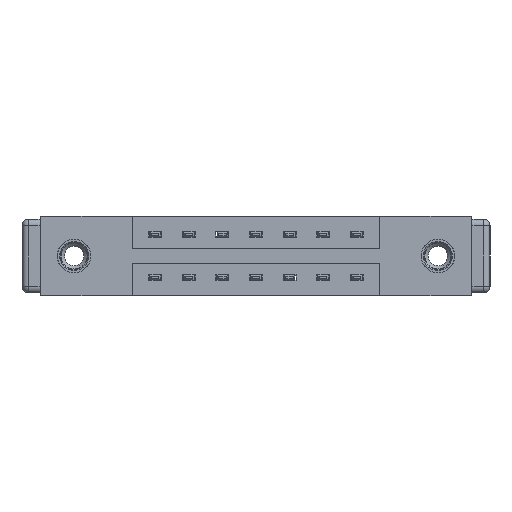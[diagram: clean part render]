
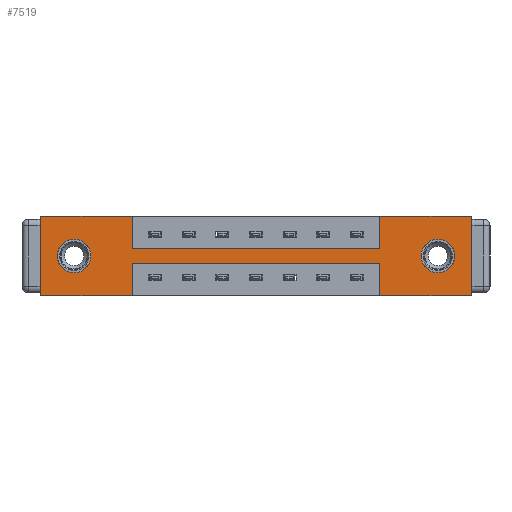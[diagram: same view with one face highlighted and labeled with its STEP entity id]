
A CAD part, front view. The second image highlights one B-rep face of the part: STEP entity #7519.
In plain terms, the highlighted planar face has unit normal (0, -1, 0).
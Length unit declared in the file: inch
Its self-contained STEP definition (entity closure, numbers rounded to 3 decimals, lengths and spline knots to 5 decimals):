
#92 = EDGE_CURVE ( 'NONE', #5666, #3161, #3983, .T. ) ;
#186 = CARTESIAN_POINT ( 'NONE',  ( 0.155, 0., -0.185 ) ) ;
#267 = CARTESIAN_POINT ( 'NONE',  ( 1.843, 0., -0.185 ) ) ;
#379 = VECTOR ( 'NONE', #10934, 39.37008 ) ;
#504 = VECTOR ( 'NONE', #2358, 39.37008 ) ;
#543 = CIRCLE ( 'NONE', #1455, 0.078 ) ;
#605 = CARTESIAN_POINT ( 'NONE',  ( 0.155, 0., -0.107 ) ) ;
#740 = CARTESIAN_POINT ( 'NONE',  ( 0., 0., 0. ) ) ;
#781 = FACE_BOUND ( 'NONE', #3398, .T. ) ;
#900 = ORIENTED_EDGE ( 'NONE', *, *, #6440, .F. ) ;
#1031 = DIRECTION ( 'NONE',  ( -1., 0., 0. ) ) ;
#1211 = DIRECTION ( 'NONE',  ( 0., 0., -1. ) ) ;
#1355 = CARTESIAN_POINT ( 'NONE',  ( 0.425, 0., -0.37 ) ) ;
#1396 = VERTEX_POINT ( 'NONE', #8295 ) ;
#1453 = CARTESIAN_POINT ( 'NONE',  ( 1.998, 0., -0.37 ) ) ;
#1455 = AXIS2_PLACEMENT_3D ( 'NONE', #186, #8013, #8932 ) ;
#1549 = EDGE_CURVE ( 'NONE', #3890, #11087, #4889, .T. ) ;
#1707 = CARTESIAN_POINT ( 'NONE',  ( 0., 0., -0.37 ) ) ;
#1768 = LINE ( 'NONE', #12552, #2092 ) ;
#1771 = DIRECTION ( 'NONE',  ( 0., 1., 0. ) ) ;
#1783 = CIRCLE ( 'NONE', #2567, 0.078 ) ;
#1805 = EDGE_CURVE ( 'NONE', #6223, #1396, #12031, .T. ) ;
#1850 = DIRECTION ( 'NONE',  ( 0., 0., -1. ) ) ;
#2052 = DIRECTION ( 'NONE',  ( 0., 0., 1. ) ) ;
#2061 = ORIENTED_EDGE ( 'NONE', *, *, #7285, .F. ) ;
#2092 = VECTOR ( 'NONE', #5840, 39.37008 ) ;
#2126 = VECTOR ( 'NONE', #8789, 39.37008 ) ;
#2205 = CARTESIAN_POINT ( 'NONE',  ( 0.425, 0., -0.37 ) ) ;
#2211 = DIRECTION ( 'NONE',  ( 0., 1., 0. ) ) ;
#2242 = EDGE_CURVE ( 'NONE', #11909, #10411, #7346, .T. ) ;
#2358 = DIRECTION ( 'NONE',  ( 0., 0., -1. ) ) ;
#2479 = LINE ( 'NONE', #7652, #12472 ) ;
#2567 = AXIS2_PLACEMENT_3D ( 'NONE', #3620, #1771, #10451 ) ;
#2671 = AXIS2_PLACEMENT_3D ( 'NONE', #267, #6084, #1211 ) ;
#2679 = AXIS2_PLACEMENT_3D ( 'NONE', #11857, #2211, #5115 ) ;
#2734 = ORIENTED_EDGE ( 'NONE', *, *, #5673, .F. ) ;
#2827 = PLANE ( 'NONE',  #10467 ) ;
#3148 = VERTEX_POINT ( 'NONE', #11028 ) ;
#3161 = VERTEX_POINT ( 'NONE', #1453 ) ;
#3244 = CARTESIAN_POINT ( 'NONE',  ( 0., 0., 0. ) ) ;
#3254 = LINE ( 'NONE', #8975, #8152 ) ;
#3398 = EDGE_LOOP ( 'NONE', ( #8268, #8948 ) ) ;
#3434 = LINE ( 'NONE', #6838, #6486 ) ;
#3491 = CARTESIAN_POINT ( 'NONE',  ( 0.425, 0., -0.22 ) ) ;
#3609 = ORIENTED_EDGE ( 'NONE', *, *, #4107, .F. ) ;
#3620 = CARTESIAN_POINT ( 'NONE',  ( 0.155, 0., -0.185 ) ) ;
#3704 = LINE ( 'NONE', #9032, #11931 ) ;
#3890 = VERTEX_POINT ( 'NONE', #3244 ) ;
#3904 = CARTESIAN_POINT ( 'NONE',  ( 0.425, 0., -0.22 ) ) ;
#3905 = CARTESIAN_POINT ( 'NONE',  ( 0.155, 0., -0.263 ) ) ;
#3983 = LINE ( 'NONE', #12521, #8166 ) ;
#4000 = ORIENTED_EDGE ( 'NONE', *, *, #8756, .T. ) ;
#4049 = DIRECTION ( 'NONE',  ( 1., 0., 0. ) ) ;
#4081 = CARTESIAN_POINT ( 'NONE',  ( 0., 0., 0. ) ) ;
#4107 = EDGE_CURVE ( 'NONE', #8267, #11909, #1768, .T. ) ;
#4152 = VERTEX_POINT ( 'NONE', #2205 ) ;
#4347 = CARTESIAN_POINT ( 'NONE',  ( 0., 0., -0.37 ) ) ;
#4491 = CARTESIAN_POINT ( 'NONE',  ( 1.573, 0., -0.37 ) ) ;
#4600 = VECTOR ( 'NONE', #5973, 39.37008 ) ;
#4695 = DIRECTION ( 'NONE',  ( 0., -1., 0. ) ) ;
#4750 = LINE ( 'NONE', #4347, #7074 ) ;
#4889 = LINE ( 'NONE', #740, #5209 ) ;
#4928 = EDGE_CURVE ( 'NONE', #3148, #7230, #3254, .T. ) ;
#4939 = EDGE_CURVE ( 'NONE', #9999, #12158, #543, .T. ) ;
#5067 = CARTESIAN_POINT ( 'NONE',  ( 1.843, 0., -0.263 ) ) ;
#5100 = EDGE_LOOP ( 'NONE', ( #4000, #6715 ) ) ;
#5115 = DIRECTION ( 'NONE',  ( 0., 0., -1. ) ) ;
#5209 = VECTOR ( 'NONE', #12365, 39.37008 ) ;
#5315 = CIRCLE ( 'NONE', #2671, 0.078 ) ;
#5433 = ORIENTED_EDGE ( 'NONE', *, *, #7022, .F. ) ;
#5452 = EDGE_CURVE ( 'NONE', #8420, #3148, #3704, .T. ) ;
#5504 = FACE_BOUND ( 'NONE', #5100, .T. ) ;
#5559 = DIRECTION ( 'NONE',  ( 0., 0., 1. ) ) ;
#5666 = VERTEX_POINT ( 'NONE', #11694 ) ;
#5673 = EDGE_CURVE ( 'NONE', #4152, #6471, #3434, .T. ) ;
#5704 = ORIENTED_EDGE ( 'NONE', *, *, #92, .F. ) ;
#5840 = DIRECTION ( 'NONE',  ( 0., 0., 1. ) ) ;
#5973 = DIRECTION ( 'NONE',  ( 0., 0., -1. ) ) ;
#6084 = DIRECTION ( 'NONE',  ( 0., 1., 0. ) ) ;
#6223 = VERTEX_POINT ( 'NONE', #5067 ) ;
#6242 = EDGE_CURVE ( 'NONE', #11087, #8420, #8298, .T. ) ;
#6392 = DIRECTION ( 'NONE',  ( -1., 0., 0. ) ) ;
#6440 = EDGE_CURVE ( 'NONE', #3161, #8267, #4750, .T. ) ;
#6471 = VERTEX_POINT ( 'NONE', #8361 ) ;
#6486 = VECTOR ( 'NONE', #1031, 39.37008 ) ;
#6598 = EDGE_LOOP ( 'NONE', ( #2061, #8880, #3609, #900, #5704, #7442, #7481, #11260, #7884, #9524, #5433, #2734 ) ) ;
#6633 = EDGE_CURVE ( 'NONE', #7230, #5666, #10709, .T. ) ;
#6715 = ORIENTED_EDGE ( 'NONE', *, *, #1805, .T. ) ;
#6838 = CARTESIAN_POINT ( 'NONE',  ( 0., 0., -0.37 ) ) ;
#7022 = EDGE_CURVE ( 'NONE', #6471, #3890, #2479, .T. ) ;
#7074 = VECTOR ( 'NONE', #6392, 39.37008 ) ;
#7214 = CARTESIAN_POINT ( 'NONE',  ( 1.573, 0., -0.22 ) ) ;
#7230 = VERTEX_POINT ( 'NONE', #8081 ) ;
#7285 = EDGE_CURVE ( 'NONE', #10411, #4152, #11155, .T. ) ;
#7346 = LINE ( 'NONE', #3904, #2126 ) ;
#7442 = ORIENTED_EDGE ( 'NONE', *, *, #6633, .F. ) ;
#7481 = ORIENTED_EDGE ( 'NONE', *, *, #4928, .F. ) ;
#7519 = ADVANCED_FACE ( 'NONE', ( #5504, #781, #8702 ), #2827, .T. ) ;
#7647 = CARTESIAN_POINT ( 'NONE',  ( 0.425, 0., 0. ) ) ;
#7652 = CARTESIAN_POINT ( 'NONE',  ( 0., 0., 0. ) ) ;
#7884 = ORIENTED_EDGE ( 'NONE', *, *, #6242, .F. ) ;
#8013 = DIRECTION ( 'NONE',  ( 0., 1., 0. ) ) ;
#8081 = CARTESIAN_POINT ( 'NONE',  ( 1.573, 0., 0. ) ) ;
#8152 = VECTOR ( 'NONE', #2052, 39.37008 ) ;
#8166 = VECTOR ( 'NONE', #1850, 39.37008 ) ;
#8267 = VERTEX_POINT ( 'NONE', #4491 ) ;
#8268 = ORIENTED_EDGE ( 'NONE', *, *, #4939, .T. ) ;
#8295 = CARTESIAN_POINT ( 'NONE',  ( 1.843, 0., -0.107 ) ) ;
#8298 = LINE ( 'NONE', #11854, #4600 ) ;
#8361 = CARTESIAN_POINT ( 'NONE',  ( 0., 0., -0.37 ) ) ;
#8380 = EDGE_CURVE ( 'NONE', #12158, #9999, #1783, .T. ) ;
#8420 = VERTEX_POINT ( 'NONE', #8647 ) ;
#8583 = DIRECTION ( 'NONE',  ( 0., 0., -1. ) ) ;
#8647 = CARTESIAN_POINT ( 'NONE',  ( 0.425, 0., -0.15 ) ) ;
#8702 = FACE_OUTER_BOUND ( 'NONE', #6598, .T. ) ;
#8756 = EDGE_CURVE ( 'NONE', #1396, #6223, #5315, .T. ) ;
#8789 = DIRECTION ( 'NONE',  ( -1., 0., 0. ) ) ;
#8880 = ORIENTED_EDGE ( 'NONE', *, *, #2242, .F. ) ;
#8932 = DIRECTION ( 'NONE',  ( 0., 0., 1. ) ) ;
#8948 = ORIENTED_EDGE ( 'NONE', *, *, #8380, .T. ) ;
#8975 = CARTESIAN_POINT ( 'NONE',  ( 1.573, 0., 0. ) ) ;
#9032 = CARTESIAN_POINT ( 'NONE',  ( 0.425, 0., -0.15 ) ) ;
#9524 = ORIENTED_EDGE ( 'NONE', *, *, #1549, .F. ) ;
#9999 = VERTEX_POINT ( 'NONE', #605 ) ;
#10411 = VERTEX_POINT ( 'NONE', #3491 ) ;
#10451 = DIRECTION ( 'NONE',  ( 0., 0., 1. ) ) ;
#10467 = AXIS2_PLACEMENT_3D ( 'NONE', #1707, #4695, #8583 ) ;
#10709 = LINE ( 'NONE', #4081, #379 ) ;
#10934 = DIRECTION ( 'NONE',  ( 1., 0., 0. ) ) ;
#11028 = CARTESIAN_POINT ( 'NONE',  ( 1.573, 0., -0.15 ) ) ;
#11087 = VERTEX_POINT ( 'NONE', #7647 ) ;
#11155 = LINE ( 'NONE', #1355, #504 ) ;
#11260 = ORIENTED_EDGE ( 'NONE', *, *, #5452, .F. ) ;
#11694 = CARTESIAN_POINT ( 'NONE',  ( 1.998, 0., 0. ) ) ;
#11854 = CARTESIAN_POINT ( 'NONE',  ( 0.425, 0., 0. ) ) ;
#11857 = CARTESIAN_POINT ( 'NONE',  ( 1.843, 0., -0.185 ) ) ;
#11909 = VERTEX_POINT ( 'NONE', #7214 ) ;
#11931 = VECTOR ( 'NONE', #4049, 39.37008 ) ;
#12031 = CIRCLE ( 'NONE', #2679, 0.078 ) ;
#12158 = VERTEX_POINT ( 'NONE', #3905 ) ;
#12365 = DIRECTION ( 'NONE',  ( 1., 0., 0. ) ) ;
#12472 = VECTOR ( 'NONE', #5559, 39.37008 ) ;
#12521 = CARTESIAN_POINT ( 'NONE',  ( 1.998, 0., 0. ) ) ;
#12552 = CARTESIAN_POINT ( 'NONE',  ( 1.573, 0., -0.37 ) ) ;
